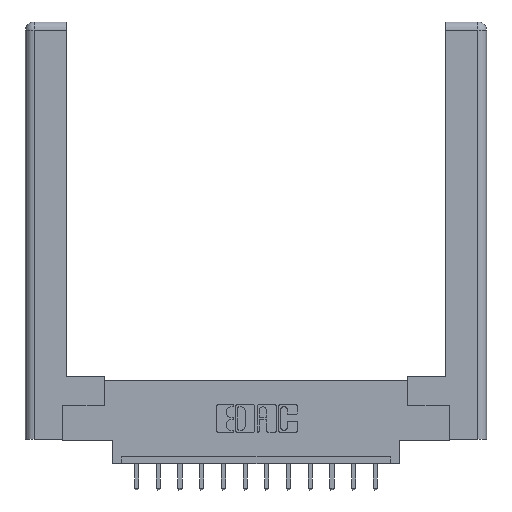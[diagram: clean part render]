
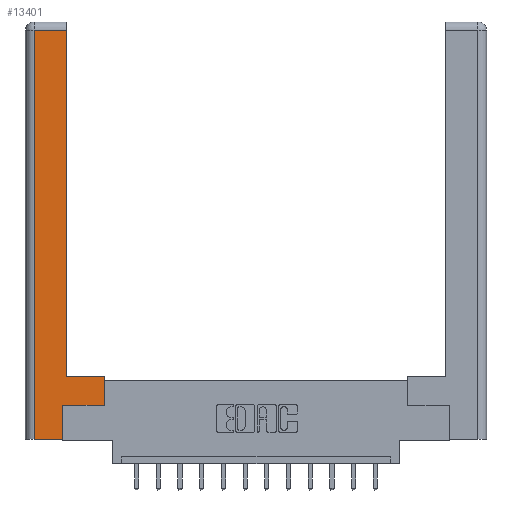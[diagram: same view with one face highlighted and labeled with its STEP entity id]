
A CAD part, top view. The second image highlights one B-rep face of the part: STEP entity #13401.
In plain terms, the highlighted planar face has unit normal (0, 0, 1).
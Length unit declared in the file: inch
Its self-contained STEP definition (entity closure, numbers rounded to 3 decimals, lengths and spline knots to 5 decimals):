
#469 = VECTOR ( 'NONE', #13758, 39.37008 ) ;
#744 = CARTESIAN_POINT ( 'NONE',  ( 0.265, 0.245, 0. ) ) ;
#815 = LINE ( 'NONE', #5343, #13306 ) ;
#1220 = CARTESIAN_POINT ( 'NONE',  ( 0.265, 0.245, 0. ) ) ;
#1225 = EDGE_CURVE ( 'NONE', #12207, #6599, #14677, .T. ) ;
#1308 = LINE ( 'NONE', #14173, #9672 ) ;
#1676 = CARTESIAN_POINT ( 'NONE',  ( 0.565, 0.245, 0. ) ) ;
#1739 = VERTEX_POINT ( 'NONE', #744 ) ;
#1985 = CARTESIAN_POINT ( 'NONE',  ( 0., 0., 0. ) ) ;
#2053 = EDGE_CURVE ( 'NONE', #1739, #9348, #815, .T. ) ;
#2130 = DIRECTION ( 'NONE',  ( -1., 0., 0. ) ) ;
#2142 = DIRECTION ( 'NONE',  ( -1., 0., 0. ) ) ;
#2321 = CARTESIAN_POINT ( 'NONE',  ( 0.295, 3., 0. ) ) ;
#2490 = ORIENTED_EDGE ( 'NONE', *, *, #3166, .T. ) ;
#2971 = EDGE_LOOP ( 'NONE', ( #8707, #13081, #5664, #5104, #2490, #8543, #13865, #3183 ) ) ;
#3105 = LINE ( 'NONE', #2321, #12922 ) ;
#3166 = EDGE_CURVE ( 'NONE', #11045, #1739, #14426, .T. ) ;
#3183 = ORIENTED_EDGE ( 'NONE', *, *, #4548, .T. ) ;
#3627 = AXIS2_PLACEMENT_3D ( 'NONE', #1985, #12854, #2142 ) ;
#4465 = CARTESIAN_POINT ( 'NONE',  ( 0.295, 0.45, 0. ) ) ;
#4523 = CARTESIAN_POINT ( 'NONE',  ( 0.0615, 0., 0. ) ) ;
#4548 = EDGE_CURVE ( 'NONE', #10408, #13771, #1308, .T. ) ;
#5104 = ORIENTED_EDGE ( 'NONE', *, *, #14897, .T. ) ;
#5343 = CARTESIAN_POINT ( 'NONE',  ( 0.565, 0.245, 0. ) ) ;
#5381 = CARTESIAN_POINT ( 'NONE',  ( 0.265, 0., 0. ) ) ;
#5477 = VECTOR ( 'NONE', #13798, 39.37008 ) ;
#5503 = CARTESIAN_POINT ( 'NONE',  ( 0.565, 0.45, 0. ) ) ;
#5664 = ORIENTED_EDGE ( 'NONE', *, *, #13730, .T. ) ;
#6599 = VERTEX_POINT ( 'NONE', #13620 ) ;
#6929 = CARTESIAN_POINT ( 'NONE',  ( 0.265, 0., 0. ) ) ;
#7308 = LINE ( 'NONE', #12710, #10686 ) ;
#8154 = EDGE_CURVE ( 'NONE', #13771, #12207, #3105, .T. ) ;
#8225 = VECTOR ( 'NONE', #13207, 39.37008 ) ;
#8543 = ORIENTED_EDGE ( 'NONE', *, *, #2053, .T. ) ;
#8608 = CARTESIAN_POINT ( 'NONE',  ( 0.0615, 0., 0. ) ) ;
#8707 = ORIENTED_EDGE ( 'NONE', *, *, #8154, .T. ) ;
#8719 = LINE ( 'NONE', #5381, #5477 ) ;
#8944 = FACE_OUTER_BOUND ( 'NONE', #2971, .T. ) ;
#9118 = CARTESIAN_POINT ( 'NONE',  ( 0.0615, 2.94, 0. ) ) ;
#9348 = VERTEX_POINT ( 'NONE', #1676 ) ;
#9474 = DIRECTION ( 'NONE',  ( 0., 1., 0. ) ) ;
#9672 = VECTOR ( 'NONE', #2130, 39.37008 ) ;
#9683 = VECTOR ( 'NONE', #14214, 39.37008 ) ;
#10408 = VERTEX_POINT ( 'NONE', #5503 ) ;
#10430 = LINE ( 'NONE', #4523, #9683 ) ;
#10439 = EDGE_CURVE ( 'NONE', #9348, #10408, #7308, .T. ) ;
#10686 = VECTOR ( 'NONE', #14943, 39.37008 ) ;
#11045 = VERTEX_POINT ( 'NONE', #6929 ) ;
#11415 = DIRECTION ( 'NONE',  ( 1., 0., 0. ) ) ;
#12207 = VERTEX_POINT ( 'NONE', #13464 ) ;
#12710 = CARTESIAN_POINT ( 'NONE',  ( 0.565, 0.45, 0. ) ) ;
#12854 = DIRECTION ( 'NONE',  ( 0., 0., -1. ) ) ;
#12922 = VECTOR ( 'NONE', #9474, 39.37008 ) ;
#13081 = ORIENTED_EDGE ( 'NONE', *, *, #1225, .T. ) ;
#13207 = DIRECTION ( 'NONE',  ( 0., 1., 0. ) ) ;
#13220 = VERTEX_POINT ( 'NONE', #8608 ) ;
#13306 = VECTOR ( 'NONE', #11415, 39.37008 ) ;
#13401 = ADVANCED_FACE ( 'NONE', ( #8944 ), #15355, .F. ) ;
#13464 = CARTESIAN_POINT ( 'NONE',  ( 0.295, 2.94, 0. ) ) ;
#13620 = CARTESIAN_POINT ( 'NONE',  ( 0.0615, 2.94, 0. ) ) ;
#13730 = EDGE_CURVE ( 'NONE', #6599, #13220, #10430, .T. ) ;
#13758 = DIRECTION ( 'NONE',  ( -1., 0., 0. ) ) ;
#13771 = VERTEX_POINT ( 'NONE', #4465 ) ;
#13798 = DIRECTION ( 'NONE',  ( 1., 0., 0. ) ) ;
#13865 = ORIENTED_EDGE ( 'NONE', *, *, #10439, .T. ) ;
#14173 = CARTESIAN_POINT ( 'NONE',  ( 0.295, 0.45, 0. ) ) ;
#14214 = DIRECTION ( 'NONE',  ( 0., -1., 0. ) ) ;
#14426 = LINE ( 'NONE', #1220, #8225 ) ;
#14677 = LINE ( 'NONE', #9118, #469 ) ;
#14897 = EDGE_CURVE ( 'NONE', #13220, #11045, #8719, .T. ) ;
#14943 = DIRECTION ( 'NONE',  ( 0., 1., 0. ) ) ;
#15355 = PLANE ( 'NONE',  #3627 ) ;
